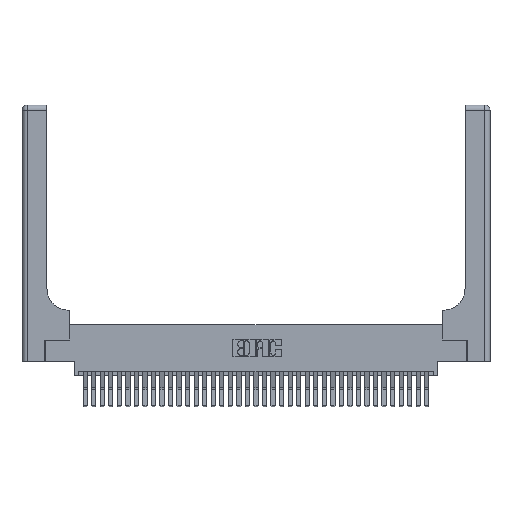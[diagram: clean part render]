
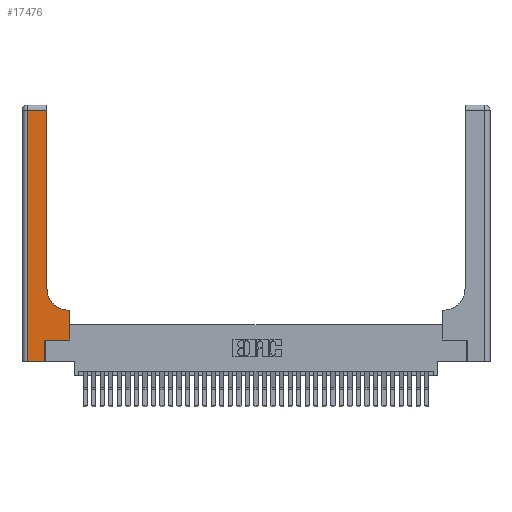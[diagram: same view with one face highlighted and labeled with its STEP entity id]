
A CAD part, top view. The second image highlights one B-rep face of the part: STEP entity #17476.
In plain terms, the highlighted planar face has unit normal (0, 0, 1).
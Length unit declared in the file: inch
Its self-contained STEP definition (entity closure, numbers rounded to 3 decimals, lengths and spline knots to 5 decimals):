
#87 = VERTEX_POINT ( 'NONE', #10192 ) ;
#89 = ORIENTED_EDGE ( 'NONE', *, *, #8348, .T. ) ;
#631 = ORIENTED_EDGE ( 'NONE', *, *, #17853, .T. ) ;
#1211 = CARTESIAN_POINT ( 'NONE',  ( 0.269, 0.25, 0.37 ) ) ;
#3139 = DIRECTION ( 'NONE',  ( -1., 0., 0. ) ) ;
#3148 = ORIENTED_EDGE ( 'NONE', *, *, #12192, .T. ) ;
#3320 = VECTOR ( 'NONE', #14542, 39.37008 ) ;
#3367 = VECTOR ( 'NONE', #35310, 39.37008 ) ;
#4099 = AXIS2_PLACEMENT_3D ( 'NONE', #12690, #33019, #15636 ) ;
#4902 = ORIENTED_EDGE ( 'NONE', *, *, #36466, .T. ) ;
#5159 = LINE ( 'NONE', #24966, #27509 ) ;
#5267 = VERTEX_POINT ( 'NONE', #11256 ) ;
#5335 = ORIENTED_EDGE ( 'NONE', *, *, #24750, .T. ) ;
#5730 = CARTESIAN_POINT ( 'NONE',  ( 0.2915, 3., 0.37 ) ) ;
#5903 = VERTEX_POINT ( 'NONE', #26409 ) ;
#6929 = LINE ( 'NONE', #10287, #7842 ) ;
#7109 = CARTESIAN_POINT ( 'NONE',  ( 0.269, 0., 0.37 ) ) ;
#7734 = CARTESIAN_POINT ( 'NONE',  ( 0.06, 2.94, 0.37 ) ) ;
#7842 = VECTOR ( 'NONE', #13234, 39.37008 ) ;
#8325 = VERTEX_POINT ( 'NONE', #23101 ) ;
#8348 = EDGE_CURVE ( 'NONE', #87, #29260, #31447, .T. ) ;
#8741 = LINE ( 'NONE', #7109, #24314 ) ;
#9766 = ORIENTED_EDGE ( 'NONE', *, *, #24689, .T. ) ;
#10192 = CARTESIAN_POINT ( 'NONE',  ( 0.2915, 0.85, 0.37 ) ) ;
#10287 = CARTESIAN_POINT ( 'NONE',  ( 0.06, 3., 0.37 ) ) ;
#11157 = LINE ( 'NONE', #17832, #3367 ) ;
#11256 = CARTESIAN_POINT ( 'NONE',  ( 0.5585, 0.25, 0.37 ) ) ;
#11652 = EDGE_LOOP ( 'NONE', ( #89, #4902, #5335, #631, #9766, #36521, #3148, #17426, #36253 ) ) ;
#12192 = EDGE_CURVE ( 'NONE', #5267, #5903, #11157, .T. ) ;
#12690 = CARTESIAN_POINT ( 'NONE',  ( 0.5415, 0.85, 0.37 ) ) ;
#12763 = LINE ( 'NONE', #13785, #35014 ) ;
#13234 = DIRECTION ( 'NONE',  ( 0., -1., 0. ) ) ;
#13785 = CARTESIAN_POINT ( 'NONE',  ( 0., 2.94, 0.37 ) ) ;
#14542 = DIRECTION ( 'NONE',  ( 1., 0., 0. ) ) ;
#15636 = DIRECTION ( 'NONE',  ( 1., 0., 0. ) ) ;
#17392 = VERTEX_POINT ( 'NONE', #20314 ) ;
#17426 = ORIENTED_EDGE ( 'NONE', *, *, #33955, .T. ) ;
#17476 = ADVANCED_FACE ( 'NONE', ( #32523 ), #26420, .F. ) ;
#17832 = CARTESIAN_POINT ( 'NONE',  ( 0.5585, 0.25, 0.37 ) ) ;
#17853 = EDGE_CURVE ( 'NONE', #24426, #8325, #34291, .T. ) ;
#19970 = CIRCLE ( 'NONE', #4099, 0.25 ) ;
#20314 = CARTESIAN_POINT ( 'NONE',  ( 0.5415, 0.6, 0.37 ) ) ;
#20699 = DIRECTION ( 'NONE',  ( 0., 0., -1. ) ) ;
#21021 = AXIS2_PLACEMENT_3D ( 'NONE', #34967, #20699, #3139 ) ;
#21118 = VERTEX_POINT ( 'NONE', #37664 ) ;
#23101 = CARTESIAN_POINT ( 'NONE',  ( 0.269, 0., 0.37 ) ) ;
#24210 = LINE ( 'NONE', #1211, #30983 ) ;
#24314 = VECTOR ( 'NONE', #27522, 39.37008 ) ;
#24426 = VERTEX_POINT ( 'NONE', #34825 ) ;
#24636 = DIRECTION ( 'NONE',  ( 1., 0., 0. ) ) ;
#24689 = EDGE_CURVE ( 'NONE', #8325, #21118, #8741, .T. ) ;
#24750 = EDGE_CURVE ( 'NONE', #30618, #24426, #6929, .T. ) ;
#24966 = CARTESIAN_POINT ( 'NONE',  ( 0.2915, 0.6, 0.37 ) ) ;
#26141 = DIRECTION ( 'NONE',  ( 0., 1., 0. ) ) ;
#26409 = CARTESIAN_POINT ( 'NONE',  ( 0.5585, 0.6, 0.37 ) ) ;
#26420 = PLANE ( 'NONE',  #21021 ) ;
#27509 = VECTOR ( 'NONE', #27869, 39.37008 ) ;
#27522 = DIRECTION ( 'NONE',  ( 0., 1., 0. ) ) ;
#27869 = DIRECTION ( 'NONE',  ( -1., 0., 0. ) ) ;
#28669 = EDGE_CURVE ( 'NONE', #17392, #87, #19970, .T. ) ;
#29260 = VERTEX_POINT ( 'NONE', #32850 ) ;
#30618 = VERTEX_POINT ( 'NONE', #7734 ) ;
#30983 = VECTOR ( 'NONE', #24636, 39.37008 ) ;
#31447 = LINE ( 'NONE', #5730, #32340 ) ;
#32340 = VECTOR ( 'NONE', #26141, 39.37008 ) ;
#32523 = FACE_OUTER_BOUND ( 'NONE', #11652, .T. ) ;
#32850 = CARTESIAN_POINT ( 'NONE',  ( 0.2915, 2.94, 0.37 ) ) ;
#33019 = DIRECTION ( 'NONE',  ( 0., 0., -1. ) ) ;
#33955 = EDGE_CURVE ( 'NONE', #5903, #17392, #5159, .T. ) ;
#34067 = DIRECTION ( 'NONE',  ( -1., 0., 0. ) ) ;
#34291 = LINE ( 'NONE', #37558, #3320 ) ;
#34825 = CARTESIAN_POINT ( 'NONE',  ( 0.06, 0., 0.37 ) ) ;
#34967 = CARTESIAN_POINT ( 'NONE',  ( 0., 3., 0.37 ) ) ;
#35014 = VECTOR ( 'NONE', #34067, 39.37008 ) ;
#35310 = DIRECTION ( 'NONE',  ( 0., 1., 0. ) ) ;
#36253 = ORIENTED_EDGE ( 'NONE', *, *, #28669, .T. ) ;
#36314 = EDGE_CURVE ( 'NONE', #21118, #5267, #24210, .T. ) ;
#36466 = EDGE_CURVE ( 'NONE', #29260, #30618, #12763, .T. ) ;
#36521 = ORIENTED_EDGE ( 'NONE', *, *, #36314, .T. ) ;
#37558 = CARTESIAN_POINT ( 'NONE',  ( 0., 0., 0.37 ) ) ;
#37664 = CARTESIAN_POINT ( 'NONE',  ( 0.269, 0.25, 0.37 ) ) ;
